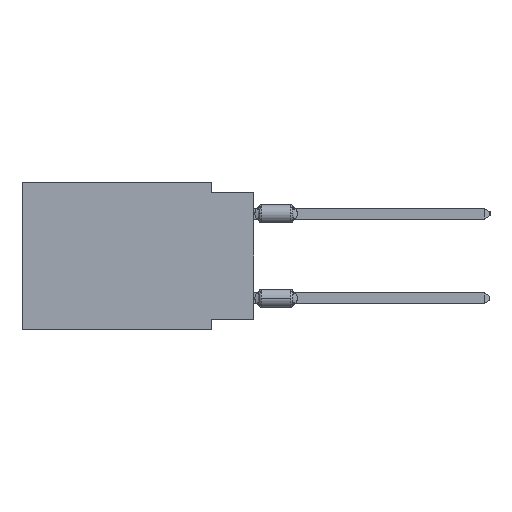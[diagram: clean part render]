
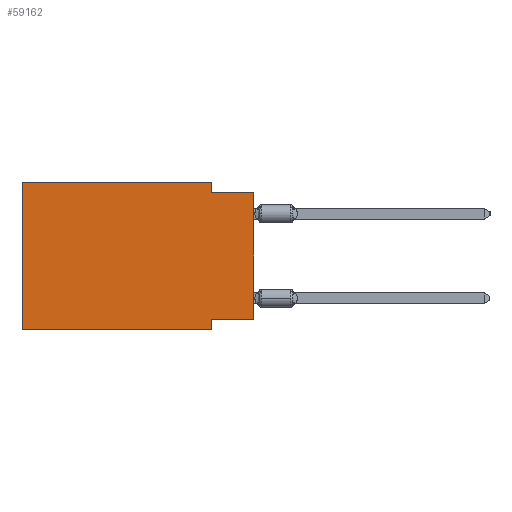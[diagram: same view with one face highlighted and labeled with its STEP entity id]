
A CAD part, left-side view. The second image highlights one B-rep face of the part: STEP entity #59162.
In plain terms, the highlighted planar face has unit normal (-1, 0, 0).
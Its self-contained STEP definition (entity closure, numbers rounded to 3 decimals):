
#87 = EDGE_CURVE ( 'NONE', #32681, #53310, #32965, .T. ) ;
#328 = EDGE_CURVE ( 'NONE', #26667, #34318, #68995, .T. ) ;
#1015 = LINE ( 'NONE', #6140, #56647 ) ;
#1962 = DIRECTION ( 'NONE',  ( 0., 0., 1. ) ) ;
#2371 = DIRECTION ( 'NONE',  ( 1., 0., 0. ) ) ;
#6140 = CARTESIAN_POINT ( 'NONE',  ( 0., 2.54, -8.89 ) ) ;
#6626 = EDGE_LOOP ( 'NONE', ( #68062, #69248, #58851, #22488, #54526, #15244, #9836, #40975 ) ) ;
#7795 = CARTESIAN_POINT ( 'NONE',  ( 0., 13.97, 0. ) ) ;
#8526 = DIRECTION ( 'NONE',  ( 0., -1., 0. ) ) ;
#9046 = VECTOR ( 'NONE', #17596, 1000. ) ;
#9836 = ORIENTED_EDGE ( 'NONE', *, *, #34719, .F. ) ;
#13721 = AXIS2_PLACEMENT_3D ( 'NONE', #40623, #2371, #46446 ) ;
#14107 = VERTEX_POINT ( 'NONE', #47203 ) ;
#15076 = LINE ( 'NONE', #59136, #57184 ) ;
#15244 = ORIENTED_EDGE ( 'NONE', *, *, #35224, .T. ) ;
#17596 = DIRECTION ( 'NONE',  ( 0., -1., 0. ) ) ;
#19945 = EDGE_CURVE ( 'NONE', #14107, #66374, #66972, .T. ) ;
#20083 = EDGE_CURVE ( 'NONE', #32681, #67099, #29464, .T. ) ;
#20201 = CARTESIAN_POINT ( 'NONE',  ( 0., 13.97, -8.89 ) ) ;
#21380 = FACE_OUTER_BOUND ( 'NONE', #6626, .T. ) ;
#22488 = ORIENTED_EDGE ( 'NONE', *, *, #39460, .F. ) ;
#23254 = CARTESIAN_POINT ( 'NONE',  ( 0., 2.54, -0.635 ) ) ;
#24740 = DIRECTION ( 'NONE',  ( 0., 1., 0. ) ) ;
#26667 = VERTEX_POINT ( 'NONE', #35379 ) ;
#28352 = DIRECTION ( 'NONE',  ( 0., 0., -1. ) ) ;
#29464 = LINE ( 'NONE', #46206, #54756 ) ;
#31064 = VERTEX_POINT ( 'NONE', #63210 ) ;
#32681 = VERTEX_POINT ( 'NONE', #39566 ) ;
#32965 = LINE ( 'NONE', #71582, #60255 ) ;
#33477 = DIRECTION ( 'NONE',  ( 0., 0., -1. ) ) ;
#34318 = VERTEX_POINT ( 'NONE', #58973 ) ;
#34685 = LINE ( 'NONE', #67474, #9046 ) ;
#34719 = EDGE_CURVE ( 'NONE', #67099, #31064, #1015, .T. ) ;
#35224 = EDGE_CURVE ( 'NONE', #26667, #31064, #38375, .T. ) ;
#35379 = CARTESIAN_POINT ( 'NONE',  ( 0., 13.97, -8.89 ) ) ;
#36942 = VECTOR ( 'NONE', #59153, 1000. ) ;
#38375 = LINE ( 'NONE', #20201, #36942 ) ;
#39460 = EDGE_CURVE ( 'NONE', #34318, #14107, #15076, .T. ) ;
#39566 = CARTESIAN_POINT ( 'NONE',  ( 0., 0., -8.255 ) ) ;
#40623 = CARTESIAN_POINT ( 'NONE',  ( 0., 13.97, 0. ) ) ;
#40975 = ORIENTED_EDGE ( 'NONE', *, *, #20083, .F. ) ;
#43112 = VECTOR ( 'NONE', #33477, 1000. ) ;
#43132 = CARTESIAN_POINT ( 'NONE',  ( 0., 2.54, -8.255 ) ) ;
#44424 = CARTESIAN_POINT ( 'NONE',  ( 0., 2.54, 0. ) ) ;
#46206 = CARTESIAN_POINT ( 'NONE',  ( 0., 0., -8.255 ) ) ;
#46446 = DIRECTION ( 'NONE',  ( 0., 0., -1. ) ) ;
#47203 = CARTESIAN_POINT ( 'NONE',  ( 0., 2.54, 0. ) ) ;
#49666 = EDGE_CURVE ( 'NONE', #66374, #53310, #34685, .T. ) ;
#49699 = DIRECTION ( 'NONE',  ( 0., 0., 1. ) ) ;
#53310 = VERTEX_POINT ( 'NONE', #57838 ) ;
#54526 = ORIENTED_EDGE ( 'NONE', *, *, #328, .F. ) ;
#54756 = VECTOR ( 'NONE', #24740, 1000. ) ;
#56647 = VECTOR ( 'NONE', #28352, 1000. ) ;
#57184 = VECTOR ( 'NONE', #8526, 1000. ) ;
#57838 = CARTESIAN_POINT ( 'NONE',  ( 0., 0., -0.635 ) ) ;
#57970 = VECTOR ( 'NONE', #1962, 1000. ) ;
#58851 = ORIENTED_EDGE ( 'NONE', *, *, #19945, .F. ) ;
#58973 = CARTESIAN_POINT ( 'NONE',  ( 0., 13.97, 0. ) ) ;
#59136 = CARTESIAN_POINT ( 'NONE',  ( 0., 13.97, 0. ) ) ;
#59153 = DIRECTION ( 'NONE',  ( 0., -1., 0. ) ) ;
#59162 = ADVANCED_FACE ( 'NONE', ( #21380 ), #60330, .F. ) ;
#60255 = VECTOR ( 'NONE', #49699, 1000. ) ;
#60330 = PLANE ( 'NONE',  #13721 ) ;
#63210 = CARTESIAN_POINT ( 'NONE',  ( 0., 2.54, -8.89 ) ) ;
#66374 = VERTEX_POINT ( 'NONE', #23254 ) ;
#66972 = LINE ( 'NONE', #44424, #43112 ) ;
#67099 = VERTEX_POINT ( 'NONE', #43132 ) ;
#67474 = CARTESIAN_POINT ( 'NONE',  ( 0., 0., -0.635 ) ) ;
#68062 = ORIENTED_EDGE ( 'NONE', *, *, #87, .T. ) ;
#68995 = LINE ( 'NONE', #7795, #57970 ) ;
#69248 = ORIENTED_EDGE ( 'NONE', *, *, #49666, .F. ) ;
#71582 = CARTESIAN_POINT ( 'NONE',  ( 0., 0., 0. ) ) ;
